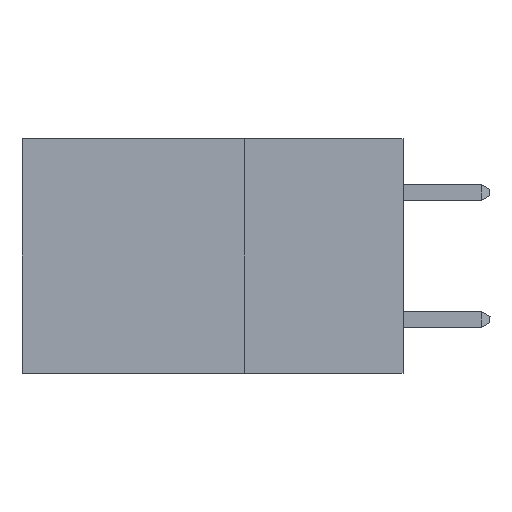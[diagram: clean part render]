
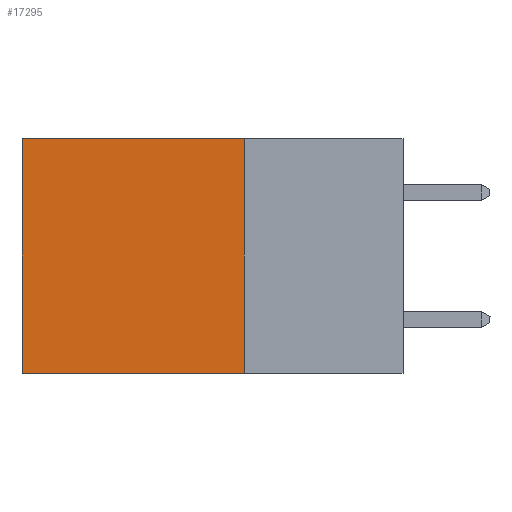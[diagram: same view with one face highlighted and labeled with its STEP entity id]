
A CAD part, left-side view. The second image highlights one B-rep face of the part: STEP entity #17295.
In plain terms, the highlighted planar face has unit normal (-1, 0, 0).
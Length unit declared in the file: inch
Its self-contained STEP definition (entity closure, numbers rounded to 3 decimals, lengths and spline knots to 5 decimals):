
#320 = CARTESIAN_POINT ( 'NONE',  ( 0.2875, 0.25, 0. ) ) ;
#1950 = DIRECTION ( 'NONE',  ( 0., 1., 0. ) ) ;
#3290 = VECTOR ( 'NONE', #31146, 39.37008 ) ;
#3534 = EDGE_LOOP ( 'NONE', ( #37770, #21735, #28021, #23767 ) ) ;
#6075 = PLANE ( 'NONE',  #40987 ) ;
#7605 = VECTOR ( 'NONE', #16512, 39.37008 ) ;
#8241 = EDGE_CURVE ( 'NONE', #42064, #37463, #28474, .T. ) ;
#9908 = CARTESIAN_POINT ( 'NONE',  ( 0.2875, 0.6, 0. ) ) ;
#10024 = CARTESIAN_POINT ( 'NONE',  ( 0.2875, 0.25, -0.37 ) ) ;
#11782 = CARTESIAN_POINT ( 'NONE',  ( 0.2875, 0.25, 0. ) ) ;
#16512 = DIRECTION ( 'NONE',  ( 0., 0., -1. ) ) ;
#17295 = ADVANCED_FACE ( 'NONE', ( #36010 ), #6075, .F. ) ;
#17411 = LINE ( 'NONE', #37501, #3290 ) ;
#18660 = VERTEX_POINT ( 'NONE', #30546 ) ;
#18859 = CARTESIAN_POINT ( 'NONE',  ( 0.2875, 0.6, 0. ) ) ;
#21735 = ORIENTED_EDGE ( 'NONE', *, *, #25717, .F. ) ;
#22848 = LINE ( 'NONE', #320, #7605 ) ;
#23087 = EDGE_CURVE ( 'NONE', #18660, #42064, #24890, .T. ) ;
#23767 = ORIENTED_EDGE ( 'NONE', *, *, #23087, .T. ) ;
#24638 = CARTESIAN_POINT ( 'NONE',  ( 0.2875, 0.6, -0.37 ) ) ;
#24890 = LINE ( 'NONE', #35160, #30941 ) ;
#25717 = EDGE_CURVE ( 'NONE', #33344, #37463, #17411, .T. ) ;
#27377 = EDGE_CURVE ( 'NONE', #18660, #33344, #22848, .T. ) ;
#28021 = ORIENTED_EDGE ( 'NONE', *, *, #27377, .F. ) ;
#28474 = LINE ( 'NONE', #18859, #40372 ) ;
#30546 = CARTESIAN_POINT ( 'NONE',  ( 0.2875, 0.25, 0. ) ) ;
#30941 = VECTOR ( 'NONE', #1950, 39.37008 ) ;
#31146 = DIRECTION ( 'NONE',  ( 0., 1., 0. ) ) ;
#33344 = VERTEX_POINT ( 'NONE', #10024 ) ;
#35154 = DIRECTION ( 'NONE',  ( 0., 0., -1. ) ) ;
#35160 = CARTESIAN_POINT ( 'NONE',  ( 0.2875, 0.25, 0. ) ) ;
#36010 = FACE_OUTER_BOUND ( 'NONE', #3534, .T. ) ;
#37463 = VERTEX_POINT ( 'NONE', #24638 ) ;
#37501 = CARTESIAN_POINT ( 'NONE',  ( 0.2875, 0.25, -0.37 ) ) ;
#37770 = ORIENTED_EDGE ( 'NONE', *, *, #8241, .T. ) ;
#38429 = DIRECTION ( 'NONE',  ( 1., 0., 0. ) ) ;
#40372 = VECTOR ( 'NONE', #41798, 39.37008 ) ;
#40987 = AXIS2_PLACEMENT_3D ( 'NONE', #11782, #38429, #35154 ) ;
#41798 = DIRECTION ( 'NONE',  ( 0., 0., -1. ) ) ;
#42064 = VERTEX_POINT ( 'NONE', #9908 ) ;
